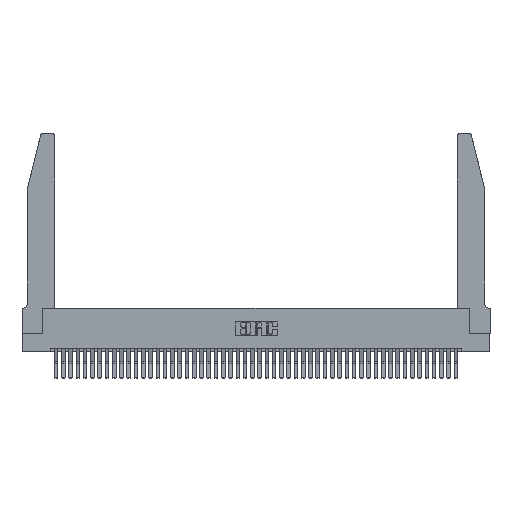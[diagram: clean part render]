
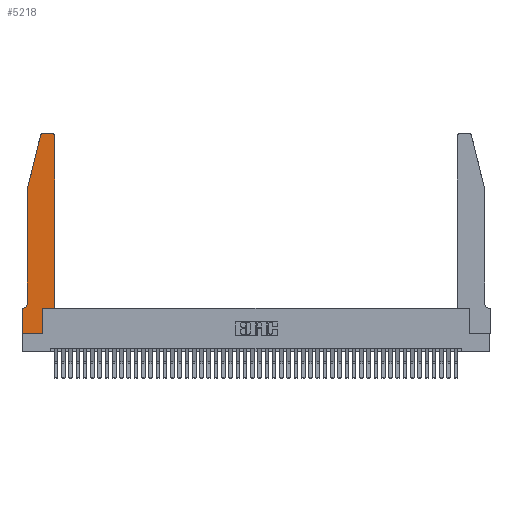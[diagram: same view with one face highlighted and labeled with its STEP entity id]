
A CAD part, top view. The second image highlights one B-rep face of the part: STEP entity #5218.
In plain terms, the highlighted planar face has unit normal (0, 0, 1).
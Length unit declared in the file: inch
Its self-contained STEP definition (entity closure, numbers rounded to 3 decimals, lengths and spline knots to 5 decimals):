
#113 = VECTOR ( 'NONE', #45983, 39.37008 ) ;
#149 = VERTEX_POINT ( 'NONE', #11158 ) ;
#350 = CARTESIAN_POINT ( 'NONE',  ( 0.25487, 2.72718, 0.37 ) ) ;
#410 = VECTOR ( 'NONE', #14841, 39.37008 ) ;
#837 = DIRECTION ( 'NONE',  ( 0., -1., 0. ) ) ;
#1871 = AXIS2_PLACEMENT_3D ( 'NONE', #32888, #11089, #36484 ) ;
#1982 = VECTOR ( 'NONE', #29686, 39.37008 ) ;
#2641 = CARTESIAN_POINT ( 'NONE',  ( 0.0755, 0.35, 0.37 ) ) ;
#2808 = EDGE_CURVE ( 'NONE', #149, #40493, #37499, .T. ) ;
#3005 = CARTESIAN_POINT ( 'NONE',  ( 0.4505, 0.35, 0.37 ) ) ;
#4189 = EDGE_CURVE ( 'NONE', #26800, #36984, #24437, .T. ) ;
#4894 = FACE_OUTER_BOUND ( 'NONE', #41867, .T. ) ;
#4988 = VECTOR ( 'NONE', #10688, 39.37008 ) ;
#5218 = ADVANCED_FACE ( 'NONE', ( #4894 ), #43097, .T. ) ;
#5287 = CIRCLE ( 'NONE', #1871, 0.03 ) ;
#7017 = LINE ( 'NONE', #26390, #44434 ) ;
#7660 = ORIENTED_EDGE ( 'NONE', *, *, #4189, .T. ) ;
#8217 = VECTOR ( 'NONE', #22193, 39.37008 ) ;
#10112 = CIRCLE ( 'NONE', #20074, 0.07 ) ;
#10688 = DIRECTION ( 'NONE',  ( 0., 1., 0. ) ) ;
#10978 = VERTEX_POINT ( 'NONE', #29194 ) ;
#10982 = DIRECTION ( 'NONE',  ( -1., 0., 0. ) ) ;
#11089 = DIRECTION ( 'NONE',  ( 0., 0., 1. ) ) ;
#11146 = CARTESIAN_POINT ( 'NONE',  ( 0.0755, 2., 0.37 ) ) ;
#11158 = CARTESIAN_POINT ( 'NONE',  ( 0.0055, 0.35, 0.37 ) ) ;
#11595 = EDGE_CURVE ( 'NONE', #40834, #21140, #33633, .T. ) ;
#12775 = ORIENTED_EDGE ( 'NONE', *, *, #35813, .T. ) ;
#13196 = VECTOR ( 'NONE', #10982, 39.37008 ) ;
#13322 = EDGE_CURVE ( 'NONE', #24412, #15522, #40159, .T. ) ;
#13571 = AXIS2_PLACEMENT_3D ( 'NONE', #42488, #20907, #46089 ) ;
#13963 = ORIENTED_EDGE ( 'NONE', *, *, #24270, .T. ) ;
#14227 = DIRECTION ( 'NONE',  ( 0., 0., -1. ) ) ;
#14841 = DIRECTION ( 'NONE',  ( -0.239, -0.971, 0. ) ) ;
#15522 = VERTEX_POINT ( 'NONE', #19185 ) ;
#15669 = ORIENTED_EDGE ( 'NONE', *, *, #32978, .T. ) ;
#16798 = EDGE_CURVE ( 'NONE', #15522, #41571, #7017, .T. ) ;
#18570 = CARTESIAN_POINT ( 'NONE',  ( 0., 0., 0.37 ) ) ;
#18892 = LINE ( 'NONE', #46773, #21150 ) ;
#19185 = CARTESIAN_POINT ( 'NONE',  ( 0.0755, 2., 0.37 ) ) ;
#20074 = AXIS2_PLACEMENT_3D ( 'NONE', #35926, #14227, #39511 ) ;
#20677 = VECTOR ( 'NONE', #28188, 39.37008 ) ;
#20818 = ORIENTED_EDGE ( 'NONE', *, *, #11595, .T. ) ;
#20907 = DIRECTION ( 'NONE',  ( 0., 0., 1. ) ) ;
#21140 = VERTEX_POINT ( 'NONE', #29366 ) ;
#21150 = VECTOR ( 'NONE', #25266, 39.37008 ) ;
#21422 = ORIENTED_EDGE ( 'NONE', *, *, #44718, .T. ) ;
#21510 = CARTESIAN_POINT ( 'NONE',  ( 0., 0.35, 0.37 ) ) ;
#22193 = DIRECTION ( 'NONE',  ( 1., 0., 0. ) ) ;
#23398 = CARTESIAN_POINT ( 'NONE',  ( 0.4205, 2.75, 0.37 ) ) ;
#24270 = EDGE_CURVE ( 'NONE', #10978, #43297, #18892, .T. ) ;
#24412 = VERTEX_POINT ( 'NONE', #350 ) ;
#24437 = LINE ( 'NONE', #28857, #4988 ) ;
#24462 = CARTESIAN_POINT ( 'NONE',  ( 0., 0., 0.37 ) ) ;
#25185 = DIRECTION ( 'NONE',  ( 1., 0., 0. ) ) ;
#25266 = DIRECTION ( 'NONE',  ( 0., 1., 0. ) ) ;
#25480 = CARTESIAN_POINT ( 'NONE',  ( 0.2605, 2.75, 0.37 ) ) ;
#26390 = CARTESIAN_POINT ( 'NONE',  ( 0.0755, 2., 0.37 ) ) ;
#26800 = VERTEX_POINT ( 'NONE', #3005 ) ;
#27487 = ORIENTED_EDGE ( 'NONE', *, *, #13322, .T. ) ;
#27578 = ORIENTED_EDGE ( 'NONE', *, *, #2808, .T. ) ;
#28170 = ORIENTED_EDGE ( 'NONE', *, *, #39703, .T. ) ;
#28188 = DIRECTION ( 'NONE',  ( -1., 0., 0. ) ) ;
#28812 = LINE ( 'NONE', #40473, #1982 ) ;
#28857 = CARTESIAN_POINT ( 'NONE',  ( 0.4505, 0.35, 0.37 ) ) ;
#29194 = CARTESIAN_POINT ( 'NONE',  ( 0.2865, 0., 0.37 ) ) ;
#29366 = CARTESIAN_POINT ( 'NONE',  ( 0.284, 2.75, 0.37 ) ) ;
#29686 = DIRECTION ( 'NONE',  ( 1., 0., 0. ) ) ;
#31300 = CARTESIAN_POINT ( 'NONE',  ( 0.2865, 0.35, 0.37 ) ) ;
#32888 = CARTESIAN_POINT ( 'NONE',  ( 0.284, 2.72, 0.37 ) ) ;
#32978 = EDGE_CURVE ( 'NONE', #40493, #45146, #38796, .T. ) ;
#33633 = LINE ( 'NONE', #25480, #13196 ) ;
#34282 = AXIS2_PLACEMENT_3D ( 'NONE', #21510, #46690, #25185 ) ;
#35813 = EDGE_CURVE ( 'NONE', #41571, #149, #10112, .T. ) ;
#35926 = CARTESIAN_POINT ( 'NONE',  ( 0.0055, 0.42, 0.37 ) ) ;
#36177 = ORIENTED_EDGE ( 'NONE', *, *, #43439, .T. ) ;
#36484 = DIRECTION ( 'NONE',  ( 1., 0., 0. ) ) ;
#36984 = VERTEX_POINT ( 'NONE', #45532 ) ;
#37223 = LINE ( 'NONE', #18570, #8217 ) ;
#37499 = LINE ( 'NONE', #2641, #20677 ) ;
#38644 = CARTESIAN_POINT ( 'NONE',  ( 0.0755, 0.42, 0.37 ) ) ;
#38796 = LINE ( 'NONE', #24462, #113 ) ;
#39511 = DIRECTION ( 'NONE',  ( -1., 0., 0. ) ) ;
#39703 = EDGE_CURVE ( 'NONE', #45146, #10978, #37223, .T. ) ;
#40159 = LINE ( 'NONE', #11146, #410 ) ;
#40167 = EDGE_CURVE ( 'NONE', #36984, #40834, #46685, .T. ) ;
#40473 = CARTESIAN_POINT ( 'NONE',  ( 0.4505, 0.35, 0.37 ) ) ;
#40493 = VERTEX_POINT ( 'NONE', #44003 ) ;
#40834 = VERTEX_POINT ( 'NONE', #23398 ) ;
#41571 = VERTEX_POINT ( 'NONE', #38644 ) ;
#41867 = EDGE_LOOP ( 'NONE', ( #20818, #21422, #27487, #45586, #12775, #27578, #15669, #28170, #13963, #36177, #7660, #46275 ) ) ;
#42233 = CARTESIAN_POINT ( 'NONE',  ( 0., 0., 0.37 ) ) ;
#42488 = CARTESIAN_POINT ( 'NONE',  ( 0.4205, 2.72, 0.37 ) ) ;
#43097 = PLANE ( 'NONE',  #34282 ) ;
#43297 = VERTEX_POINT ( 'NONE', #31300 ) ;
#43439 = EDGE_CURVE ( 'NONE', #43297, #26800, #28812, .T. ) ;
#44003 = CARTESIAN_POINT ( 'NONE',  ( 0., 0.35, 0.37 ) ) ;
#44434 = VECTOR ( 'NONE', #837, 39.37008 ) ;
#44718 = EDGE_CURVE ( 'NONE', #21140, #24412, #5287, .T. ) ;
#45146 = VERTEX_POINT ( 'NONE', #42233 ) ;
#45532 = CARTESIAN_POINT ( 'NONE',  ( 0.4505, 2.72, 0.37 ) ) ;
#45586 = ORIENTED_EDGE ( 'NONE', *, *, #16798, .T. ) ;
#45983 = DIRECTION ( 'NONE',  ( 0., -1., 0. ) ) ;
#46089 = DIRECTION ( 'NONE',  ( 1., 0., 0. ) ) ;
#46275 = ORIENTED_EDGE ( 'NONE', *, *, #40167, .T. ) ;
#46685 = CIRCLE ( 'NONE', #13571, 0.03 ) ;
#46690 = DIRECTION ( 'NONE',  ( 0., 0., 1. ) ) ;
#46773 = CARTESIAN_POINT ( 'NONE',  ( 0.2865, 0.35, 0.37 ) ) ;
